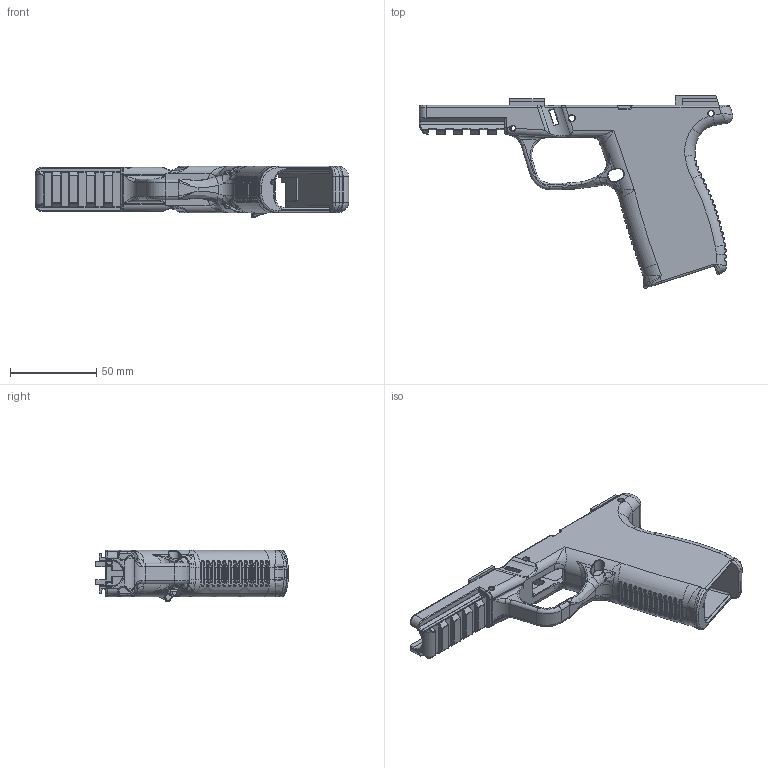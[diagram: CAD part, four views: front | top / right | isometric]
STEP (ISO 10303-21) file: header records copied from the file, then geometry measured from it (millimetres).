
FILE_DESCRIPTION(/* description */ (''),/* implementation_level */ '2;1');
FILE_NAME(/* name */ 'SW9.step',/* time_stamp */ '2021-10-26T17:42:56-04:00',/* author */ (''),/* organization */ (''),/* preprocessor_version */ 'ST-DEVELOPER v18.1',/* originating_system */ 'Autodesk Translation Framework v10.10.0.1391',/* authorisation */ '');
FILE_SCHEMA (('AUTOMOTIVE_DESIGN { 1 0 10303 214 3 1 1 }'));
Products named in the file (5): SW9; Front Rail; SW9 Module; SW Frame; Rail Spec
Assembly tree (4 placements, depth 2):
  SW9
    Front Rail
    SW9 Module
    SW Frame
    Rail Spec
Bounding box: 181.73 x 111.56 x 30 mm (x, y, z)
Volume: 94300.2 mm3; surface area: 51972 mm2
Topology: 5 solids, 5 shells, 1793 faces, 4443 edges, 2553 vertices
Faces by surface type: bspline 627, cylinder 604, plane 337, torus 184, cone 22, sphere 19
Full cylindrical faces by diameter (mm): 2.159 x1, 2.5 x1, 3.175 x3, 3.3 x5, 3.6 x2
Entity records: 74720 total; most frequent: CARTESIAN_POINT 34618, ORIENTED_EDGE 8708, DIRECTION 8049, EDGE_CURVE 4354, AXIS2_PLACEMENT_3D 3284, VERTEX_POINT 2551, EDGE_LOOP 1809, FACE_OUTER_BOUND 1793
